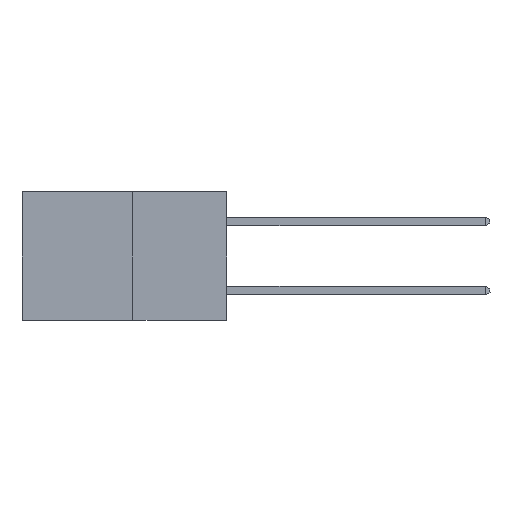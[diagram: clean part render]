
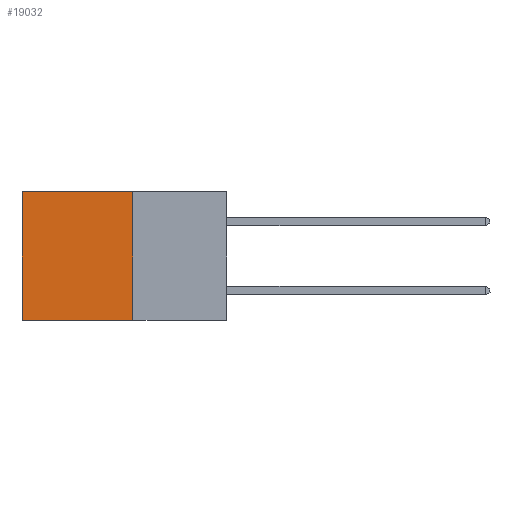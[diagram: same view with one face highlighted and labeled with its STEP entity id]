
A CAD part, left-side view. The second image highlights one B-rep face of the part: STEP entity #19032.
In plain terms, the highlighted planar face has unit normal (-1, 0, 0).
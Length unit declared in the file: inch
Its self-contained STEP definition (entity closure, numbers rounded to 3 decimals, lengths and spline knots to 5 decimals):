
#574 = CARTESIAN_POINT ( 'NONE',  ( 0.277, 0.27, -0.37 ) ) ;
#1221 = CARTESIAN_POINT ( 'NONE',  ( 0.277, 0.27, 0. ) ) ;
#1824 = CARTESIAN_POINT ( 'NONE',  ( 0.277, 0.59, -0.37 ) ) ;
#2437 = LINE ( 'NONE', #574, #6815 ) ;
#2780 = VECTOR ( 'NONE', #6546, 39.37008 ) ;
#3488 = ORIENTED_EDGE ( 'NONE', *, *, #5514, .T. ) ;
#5492 = VERTEX_POINT ( 'NONE', #24030 ) ;
#5514 = EDGE_CURVE ( 'NONE', #5492, #22608, #12965, .T. ) ;
#6546 = DIRECTION ( 'NONE',  ( 0., 1., 0. ) ) ;
#6815 = VECTOR ( 'NONE', #17422, 39.37008 ) ;
#7215 = CARTESIAN_POINT ( 'NONE',  ( 0.277, 0.59, -0.37 ) ) ;
#7740 = LINE ( 'NONE', #14004, #2780 ) ;
#8003 = CARTESIAN_POINT ( 'NONE',  ( 0.277, 0.27, 0. ) ) ;
#8588 = DIRECTION ( 'NONE',  ( 0., 0., -1. ) ) ;
#8884 = ORIENTED_EDGE ( 'NONE', *, *, #24199, .F. ) ;
#9941 = ORIENTED_EDGE ( 'NONE', *, *, #10121, .T. ) ;
#10121 = EDGE_CURVE ( 'NONE', #21554, #5492, #22129, .T. ) ;
#10816 = CARTESIAN_POINT ( 'NONE',  ( 0.277, 0.27, -0.37 ) ) ;
#11259 = EDGE_CURVE ( 'NONE', #21554, #23172, #2437, .T. ) ;
#12965 = LINE ( 'NONE', #7215, #23559 ) ;
#13943 = EDGE_LOOP ( 'NONE', ( #3488, #8884, #15249, #9941 ) ) ;
#14004 = CARTESIAN_POINT ( 'NONE',  ( 0.277, 0.27, -0.37 ) ) ;
#15249 = ORIENTED_EDGE ( 'NONE', *, *, #11259, .F. ) ;
#16335 = DIRECTION ( 'NONE',  ( 0., 1., 0. ) ) ;
#16743 = AXIS2_PLACEMENT_3D ( 'NONE', #17956, #19847, #8588 ) ;
#17152 = VECTOR ( 'NONE', #16335, 39.37008 ) ;
#17422 = DIRECTION ( 'NONE',  ( 0., 0., -1. ) ) ;
#17956 = CARTESIAN_POINT ( 'NONE',  ( 0.277, 0.27, -0.37 ) ) ;
#18979 = FACE_OUTER_BOUND ( 'NONE', #13943, .T. ) ;
#19032 = ADVANCED_FACE ( 'NONE', ( #18979 ), #23529, .F. ) ;
#19847 = DIRECTION ( 'NONE',  ( 1., 0., 0. ) ) ;
#21554 = VERTEX_POINT ( 'NONE', #8003 ) ;
#22129 = LINE ( 'NONE', #1221, #17152 ) ;
#22221 = DIRECTION ( 'NONE',  ( 0., 0., -1. ) ) ;
#22608 = VERTEX_POINT ( 'NONE', #1824 ) ;
#23172 = VERTEX_POINT ( 'NONE', #10816 ) ;
#23529 = PLANE ( 'NONE',  #16743 ) ;
#23559 = VECTOR ( 'NONE', #22221, 39.37008 ) ;
#24030 = CARTESIAN_POINT ( 'NONE',  ( 0.277, 0.59, 0. ) ) ;
#24199 = EDGE_CURVE ( 'NONE', #23172, #22608, #7740, .T. ) ;
